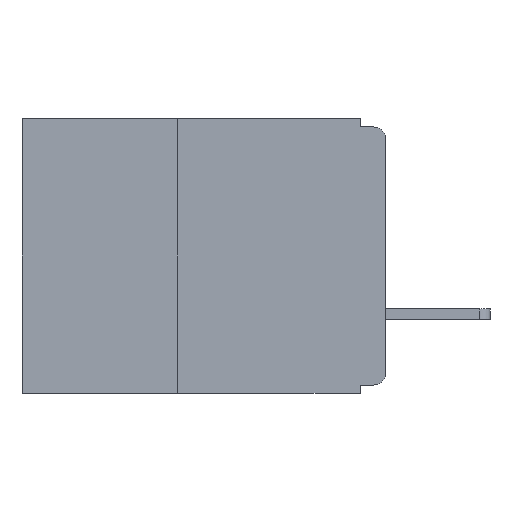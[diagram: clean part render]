
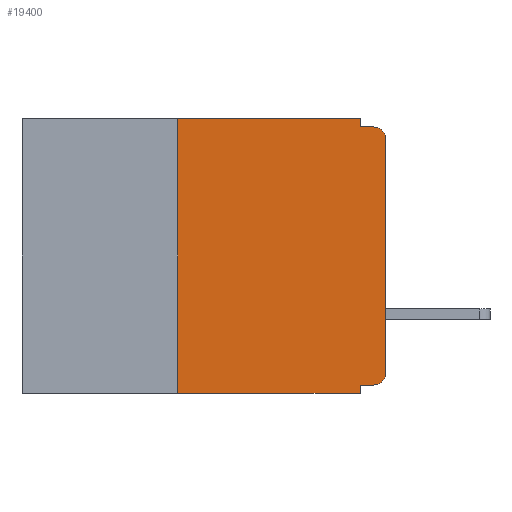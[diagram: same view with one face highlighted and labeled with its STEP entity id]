
A CAD part, left-side view. The second image highlights one B-rep face of the part: STEP entity #19400.
In plain terms, the highlighted planar face has unit normal (-1, 0, 0).
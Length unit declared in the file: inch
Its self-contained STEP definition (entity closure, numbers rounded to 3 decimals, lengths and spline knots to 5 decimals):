
#721 = LINE ( 'NONE', #28485, #20595 ) ;
#842 = CARTESIAN_POINT ( 'NONE',  ( 0., 0., -0.025 ) ) ;
#1196 = CARTESIAN_POINT ( 'NONE',  ( 0., 0.015, -0.01 ) ) ;
#1236 = VERTEX_POINT ( 'NONE', #4951 ) ;
#1401 = VERTEX_POINT ( 'NONE', #9436 ) ;
#1464 = LINE ( 'NONE', #27150, #12730 ) ;
#1489 = DIRECTION ( 'NONE',  ( 1., 0., 0. ) ) ;
#1734 = CARTESIAN_POINT ( 'NONE',  ( 0., 0.25, 0. ) ) ;
#2390 = ORIENTED_EDGE ( 'NONE', *, *, #12977, .F. ) ;
#3025 = CARTESIAN_POINT ( 'NONE',  ( 0., 0.031, 0. ) ) ;
#3285 = ORIENTED_EDGE ( 'NONE', *, *, #16276, .F. ) ;
#3522 = VERTEX_POINT ( 'NONE', #1734 ) ;
#3747 = ORIENTED_EDGE ( 'NONE', *, *, #20575, .T. ) ;
#3907 = VERTEX_POINT ( 'NONE', #25047 ) ;
#4697 = VECTOR ( 'NONE', #23903, 39.37008 ) ;
#4951 = CARTESIAN_POINT ( 'NONE',  ( 0., 0.25, -0.33 ) ) ;
#5751 = CARTESIAN_POINT ( 'NONE',  ( 0., 0.015, -0.305 ) ) ;
#5823 = VERTEX_POINT ( 'NONE', #1196 ) ;
#5837 = EDGE_CURVE ( 'NONE', #10884, #5823, #13169, .T. ) ;
#6229 = DIRECTION ( 'NONE',  ( 0., 0., -1. ) ) ;
#6449 = DIRECTION ( 'NONE',  ( 0., -1., 0. ) ) ;
#6669 = LINE ( 'NONE', #20068, #18652 ) ;
#6756 = CARTESIAN_POINT ( 'NONE',  ( 0., 0.015, -0.32 ) ) ;
#8174 = DIRECTION ( 'NONE',  ( 0., 0., -1. ) ) ;
#8459 = VERTEX_POINT ( 'NONE', #22335 ) ;
#8809 = EDGE_CURVE ( 'NONE', #1236, #1401, #9584, .T. ) ;
#8882 = CARTESIAN_POINT ( 'NONE',  ( 0., 0., -0.01 ) ) ;
#9022 = CARTESIAN_POINT ( 'NONE',  ( 0., 0., -0.32 ) ) ;
#9362 = ORIENTED_EDGE ( 'NONE', *, *, #17093, .F. ) ;
#9436 = CARTESIAN_POINT ( 'NONE',  ( 0., 0.031, -0.33 ) ) ;
#9441 = FACE_OUTER_BOUND ( 'NONE', #26201, .T. ) ;
#9584 = LINE ( 'NONE', #26633, #4697 ) ;
#9911 = AXIS2_PLACEMENT_3D ( 'NONE', #29861, #1489, #18249 ) ;
#10884 = VERTEX_POINT ( 'NONE', #842 ) ;
#12328 = DIRECTION ( 'NONE',  ( 0., -1., 0. ) ) ;
#12730 = VECTOR ( 'NONE', #29418, 39.37008 ) ;
#12977 = EDGE_CURVE ( 'NONE', #1236, #3522, #1464, .T. ) ;
#13169 = CIRCLE ( 'NONE', #24012, 0.015 ) ;
#13270 = VECTOR ( 'NONE', #12328, 39.37008 ) ;
#13588 = EDGE_CURVE ( 'NONE', #3907, #10884, #6669, .T. ) ;
#14039 = CARTESIAN_POINT ( 'NONE',  ( 0., 0.031, -0.01 ) ) ;
#14382 = DIRECTION ( 'NONE',  ( 0., 0., -1. ) ) ;
#15148 = ORIENTED_EDGE ( 'NONE', *, *, #17241, .F. ) ;
#15191 = ORIENTED_EDGE ( 'NONE', *, *, #13588, .T. ) ;
#15540 = AXIS2_PLACEMENT_3D ( 'NONE', #5751, #22480, #8174 ) ;
#16276 = EDGE_CURVE ( 'NONE', #8459, #1401, #27382, .T. ) ;
#17093 = EDGE_CURVE ( 'NONE', #27750, #5823, #24040, .T. ) ;
#17241 = EDGE_CURVE ( 'NONE', #3522, #17940, #26606, .T. ) ;
#17346 = ORIENTED_EDGE ( 'NONE', *, *, #20344, .F. ) ;
#17537 = ORIENTED_EDGE ( 'NONE', *, *, #5837, .T. ) ;
#17940 = VERTEX_POINT ( 'NONE', #3025 ) ;
#18249 = DIRECTION ( 'NONE',  ( 0., 0., -1. ) ) ;
#18618 = DIRECTION ( 'NONE',  ( 0., 1., 0. ) ) ;
#18652 = VECTOR ( 'NONE', #22436, 39.37008 ) ;
#19400 = ADVANCED_FACE ( 'NONE', ( #9441 ), #27598, .F. ) ;
#19431 = ORIENTED_EDGE ( 'NONE', *, *, #8809, .T. ) ;
#19442 = CARTESIAN_POINT ( 'NONE',  ( 0., 0.437, 0. ) ) ;
#19738 = CIRCLE ( 'NONE', #15540, 0.015 ) ;
#20068 = CARTESIAN_POINT ( 'NONE',  ( 0., 0., 0. ) ) ;
#20344 = EDGE_CURVE ( 'NONE', #17940, #27750, #721, .T. ) ;
#20575 = EDGE_CURVE ( 'NONE', #26612, #3907, #19738, .T. ) ;
#20595 = VECTOR ( 'NONE', #14382, 39.37008 ) ;
#22335 = CARTESIAN_POINT ( 'NONE',  ( 0., 0.031, -0.32 ) ) ;
#22436 = DIRECTION ( 'NONE',  ( 0., 0., 1. ) ) ;
#22480 = DIRECTION ( 'NONE',  ( -1., 0., 0. ) ) ;
#23487 = ORIENTED_EDGE ( 'NONE', *, *, #25918, .F. ) ;
#23903 = DIRECTION ( 'NONE',  ( 0., -1., 0. ) ) ;
#24012 = AXIS2_PLACEMENT_3D ( 'NONE', #30646, #30606, #30589 ) ;
#24040 = LINE ( 'NONE', #8882, #29435 ) ;
#25047 = CARTESIAN_POINT ( 'NONE',  ( 0., 0., -0.305 ) ) ;
#25172 = CARTESIAN_POINT ( 'NONE',  ( 0., 0.031, -0.33 ) ) ;
#25649 = LINE ( 'NONE', #9022, #30280 ) ;
#25918 = EDGE_CURVE ( 'NONE', #26612, #8459, #25649, .T. ) ;
#26201 = EDGE_LOOP ( 'NONE', ( #15191, #17537, #9362, #17346, #15148, #2390, #19431, #3285, #23487, #3747 ) ) ;
#26606 = LINE ( 'NONE', #19442, #13270 ) ;
#26612 = VERTEX_POINT ( 'NONE', #6756 ) ;
#26633 = CARTESIAN_POINT ( 'NONE',  ( 0., 0.437, -0.33 ) ) ;
#26663 = VECTOR ( 'NONE', #6229, 39.37008 ) ;
#27150 = CARTESIAN_POINT ( 'NONE',  ( 0., 0.25, -0.33 ) ) ;
#27382 = LINE ( 'NONE', #25172, #26663 ) ;
#27598 = PLANE ( 'NONE',  #9911 ) ;
#27750 = VERTEX_POINT ( 'NONE', #14039 ) ;
#28485 = CARTESIAN_POINT ( 'NONE',  ( 0., 0.031, 0. ) ) ;
#29418 = DIRECTION ( 'NONE',  ( 0., 0., 1. ) ) ;
#29435 = VECTOR ( 'NONE', #6449, 39.37008 ) ;
#29861 = CARTESIAN_POINT ( 'NONE',  ( 0., 0.437, 0. ) ) ;
#30280 = VECTOR ( 'NONE', #18618, 39.37008 ) ;
#30589 = DIRECTION ( 'NONE',  ( 0., 0., -1. ) ) ;
#30606 = DIRECTION ( 'NONE',  ( -1., 0., 0. ) ) ;
#30646 = CARTESIAN_POINT ( 'NONE',  ( 0., 0.015, -0.025 ) ) ;
